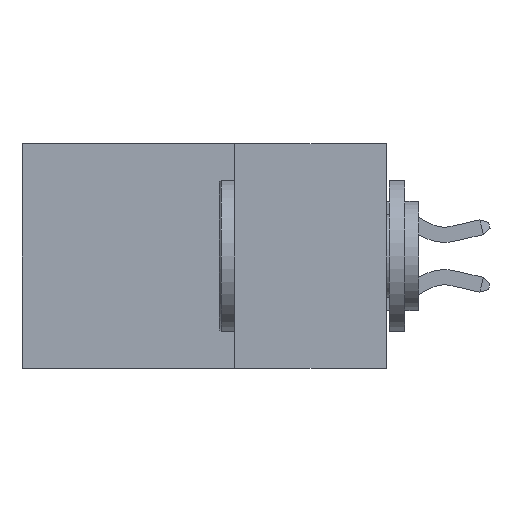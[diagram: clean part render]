
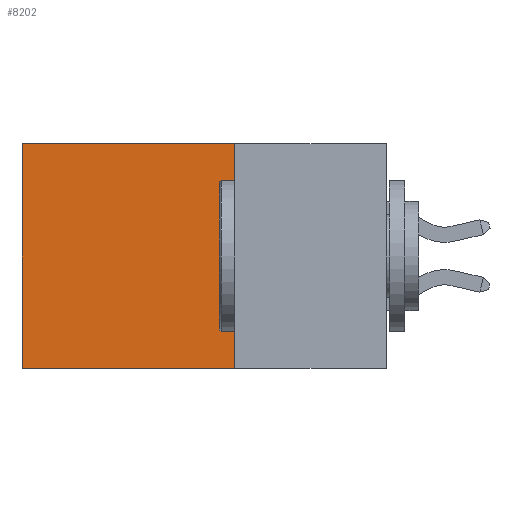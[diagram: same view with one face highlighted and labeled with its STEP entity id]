
A CAD part, left-side view. The second image highlights one B-rep face of the part: STEP entity #8202.
In plain terms, the highlighted planar face has unit normal (-1, 0, 0).
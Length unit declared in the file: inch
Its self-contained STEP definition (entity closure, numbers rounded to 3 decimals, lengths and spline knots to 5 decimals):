
#229 = ORIENTED_EDGE ( 'NONE', *, *, #8725, .F. ) ;
#430 = DIRECTION ( 'NONE',  ( 0., 0., -1. ) ) ;
#479 = AXIS2_PLACEMENT_3D ( 'NONE', #1204, #6723, #4419 ) ;
#702 = DIRECTION ( 'NONE',  ( 0., 0., -1. ) ) ;
#953 = CARTESIAN_POINT ( 'NONE',  ( 0.2615, 0.6, -0.37 ) ) ;
#1006 = LINE ( 'NONE', #8149, #10160 ) ;
#1204 = CARTESIAN_POINT ( 'NONE',  ( 0.2615, 0.25, -0.37 ) ) ;
#1723 = CARTESIAN_POINT ( 'NONE',  ( 0.2615, 0.6, 0. ) ) ;
#2257 = VECTOR ( 'NONE', #6043, 39.37008 ) ;
#2780 = CARTESIAN_POINT ( 'NONE',  ( 0.2615, 0.25, 0. ) ) ;
#3058 = CARTESIAN_POINT ( 'NONE',  ( 0.2615, 0.6, -0.37 ) ) ;
#3467 = FACE_OUTER_BOUND ( 'NONE', #6388, .T. ) ;
#3517 = VERTEX_POINT ( 'NONE', #1723 ) ;
#4105 = VECTOR ( 'NONE', #430, 39.37008 ) ;
#4301 = EDGE_CURVE ( 'NONE', #3517, #6277, #4562, .T. ) ;
#4419 = DIRECTION ( 'NONE',  ( 0., 0., -1. ) ) ;
#4562 = LINE ( 'NONE', #3058, #7849 ) ;
#4665 = CARTESIAN_POINT ( 'NONE',  ( 0.2615, 0.25, 0. ) ) ;
#5072 = EDGE_CURVE ( 'NONE', #7376, #3517, #10039, .T. ) ;
#5299 = LINE ( 'NONE', #8569, #4105 ) ;
#6043 = DIRECTION ( 'NONE',  ( 0., 1., 0. ) ) ;
#6277 = VERTEX_POINT ( 'NONE', #953 ) ;
#6290 = ORIENTED_EDGE ( 'NONE', *, *, #5072, .T. ) ;
#6388 = EDGE_LOOP ( 'NONE', ( #9915, #9644, #229, #6290 ) ) ;
#6723 = DIRECTION ( 'NONE',  ( 1., 0., 0. ) ) ;
#7376 = VERTEX_POINT ( 'NONE', #4665 ) ;
#7849 = VECTOR ( 'NONE', #702, 39.37008 ) ;
#8149 = CARTESIAN_POINT ( 'NONE',  ( 0.2615, 0.25, -0.37 ) ) ;
#8202 = ADVANCED_FACE ( 'NONE', ( #3467 ), #9143, .F. ) ;
#8250 = DIRECTION ( 'NONE',  ( 0., 1., 0. ) ) ;
#8441 = VERTEX_POINT ( 'NONE', #10417 ) ;
#8569 = CARTESIAN_POINT ( 'NONE',  ( 0.2615, 0.25, -0.37 ) ) ;
#8573 = EDGE_CURVE ( 'NONE', #8441, #6277, #1006, .T. ) ;
#8725 = EDGE_CURVE ( 'NONE', #7376, #8441, #5299, .T. ) ;
#9143 = PLANE ( 'NONE',  #479 ) ;
#9644 = ORIENTED_EDGE ( 'NONE', *, *, #8573, .F. ) ;
#9915 = ORIENTED_EDGE ( 'NONE', *, *, #4301, .T. ) ;
#10039 = LINE ( 'NONE', #2780, #2257 ) ;
#10160 = VECTOR ( 'NONE', #8250, 39.37008 ) ;
#10417 = CARTESIAN_POINT ( 'NONE',  ( 0.2615, 0.25, -0.37 ) ) ;
